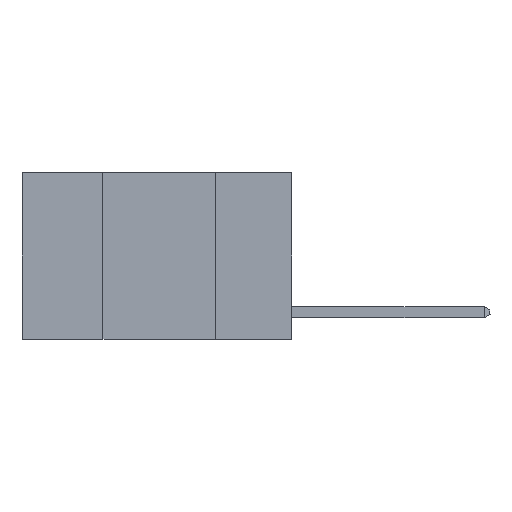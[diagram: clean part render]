
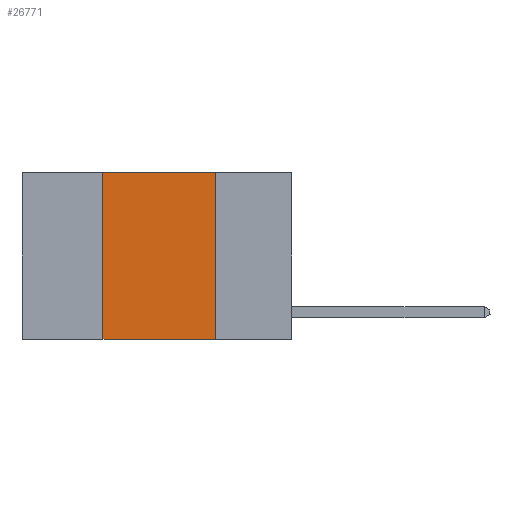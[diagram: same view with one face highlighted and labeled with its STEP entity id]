
A CAD part, left-side view. The second image highlights one B-rep face of the part: STEP entity #26771.
In plain terms, the highlighted planar face has unit normal (-1, 0, 0).
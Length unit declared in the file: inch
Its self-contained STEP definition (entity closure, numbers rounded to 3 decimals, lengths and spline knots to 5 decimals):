
#588 = EDGE_CURVE ( 'NONE', #9091, #3064, #25032, .T. ) ;
#940 = CARTESIAN_POINT ( 'NONE',  ( 0., 0.42, 0. ) ) ;
#1152 = ORIENTED_EDGE ( 'NONE', *, *, #13011, .T. ) ;
#1507 = DIRECTION ( 'NONE',  ( 0., 0., 1. ) ) ;
#2146 = VECTOR ( 'NONE', #10473, 39.37008 ) ;
#3064 = VERTEX_POINT ( 'NONE', #26692 ) ;
#3169 = VERTEX_POINT ( 'NONE', #16751 ) ;
#4857 = CARTESIAN_POINT ( 'NONE',  ( 0., 0.17, 0. ) ) ;
#5811 = LINE ( 'NONE', #23188, #7065 ) ;
#7065 = VECTOR ( 'NONE', #1507, 39.37008 ) ;
#7510 = ORIENTED_EDGE ( 'NONE', *, *, #24010, .F. ) ;
#9074 = DIRECTION ( 'NONE',  ( 0., 0., -1. ) ) ;
#9091 = VERTEX_POINT ( 'NONE', #940 ) ;
#10156 = DIRECTION ( 'NONE',  ( 0., -1., 0. ) ) ;
#10287 = LINE ( 'NONE', #14947, #12068 ) ;
#10473 = DIRECTION ( 'NONE',  ( 0., -1., 0. ) ) ;
#11277 = DIRECTION ( 'NONE',  ( 1., 0., 0. ) ) ;
#12068 = VECTOR ( 'NONE', #10156, 39.37008 ) ;
#13011 = EDGE_CURVE ( 'NONE', #3169, #24110, #10287, .T. ) ;
#13832 = ORIENTED_EDGE ( 'NONE', *, *, #23659, .F. ) ;
#14143 = CARTESIAN_POINT ( 'NONE',  ( 0., 0.6, 0. ) ) ;
#14321 = AXIS2_PLACEMENT_3D ( 'NONE', #15914, #11277, #26539 ) ;
#14947 = CARTESIAN_POINT ( 'NONE',  ( 0., 0.6, -0.37 ) ) ;
#15509 = PLANE ( 'NONE',  #14321 ) ;
#15914 = CARTESIAN_POINT ( 'NONE',  ( 0., 0.6, 0. ) ) ;
#16751 = CARTESIAN_POINT ( 'NONE',  ( 0., 0.42, -0.37 ) ) ;
#21642 = CARTESIAN_POINT ( 'NONE',  ( 0., 0.17, -0.37 ) ) ;
#21869 = EDGE_LOOP ( 'NONE', ( #13832, #22940, #7510, #1152 ) ) ;
#22688 = VECTOR ( 'NONE', #9074, 39.37008 ) ;
#22940 = ORIENTED_EDGE ( 'NONE', *, *, #588, .F. ) ;
#23188 = CARTESIAN_POINT ( 'NONE',  ( 0., 0.42, 0. ) ) ;
#23659 = EDGE_CURVE ( 'NONE', #3064, #24110, #26016, .T. ) ;
#24010 = EDGE_CURVE ( 'NONE', #3169, #9091, #5811, .T. ) ;
#24110 = VERTEX_POINT ( 'NONE', #21642 ) ;
#24438 = FACE_OUTER_BOUND ( 'NONE', #21869, .T. ) ;
#25032 = LINE ( 'NONE', #14143, #2146 ) ;
#26016 = LINE ( 'NONE', #4857, #22688 ) ;
#26539 = DIRECTION ( 'NONE',  ( 0., 0., -1. ) ) ;
#26692 = CARTESIAN_POINT ( 'NONE',  ( 0., 0.17, 0. ) ) ;
#26771 = ADVANCED_FACE ( 'NONE', ( #24438 ), #15509, .F. ) ;
